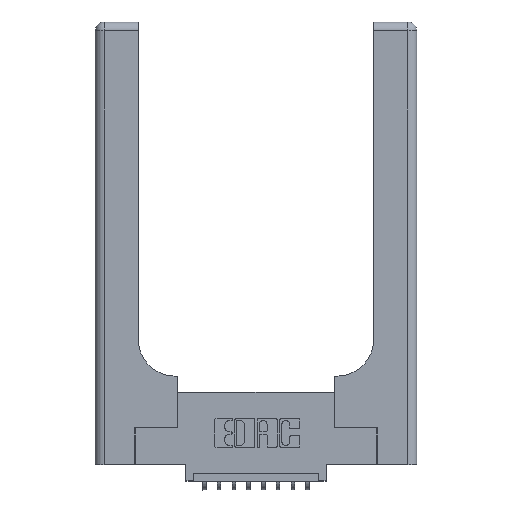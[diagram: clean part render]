
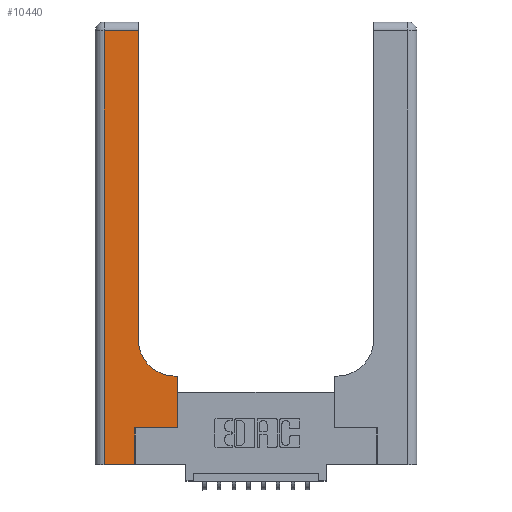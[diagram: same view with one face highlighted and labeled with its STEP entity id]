
A CAD part, top view. The second image highlights one B-rep face of the part: STEP entity #10440.
In plain terms, the highlighted planar face has unit normal (0, 0, 1).
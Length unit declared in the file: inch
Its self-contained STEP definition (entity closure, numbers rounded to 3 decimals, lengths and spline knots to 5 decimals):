
#51 = VECTOR ( 'NONE', #11838, 39.37008 ) ;
#222 = EDGE_CURVE ( 'NONE', #4829, #1192, #12432, .T. ) ;
#254 = CARTESIAN_POINT ( 'NONE',  ( 0.06, 2.94, 0.37 ) ) ;
#439 = DIRECTION ( 'NONE',  ( 0., 1., 0. ) ) ;
#472 = CIRCLE ( 'NONE', #12378, 0.25 ) ;
#584 = CARTESIAN_POINT ( 'NONE',  ( 0.269, 0.25, 0.37 ) ) ;
#1157 = ORIENTED_EDGE ( 'NONE', *, *, #15149, .T. ) ;
#1192 = VERTEX_POINT ( 'NONE', #12642 ) ;
#1278 = CARTESIAN_POINT ( 'NONE',  ( 0.269, 0., 0.37 ) ) ;
#1284 = VERTEX_POINT ( 'NONE', #8290 ) ;
#1441 = EDGE_CURVE ( 'NONE', #3802, #15325, #15326, .T. ) ;
#1727 = LINE ( 'NONE', #5273, #5572 ) ;
#1786 = CARTESIAN_POINT ( 'NONE',  ( 0.2915, 0.6, 0.37 ) ) ;
#1810 = EDGE_LOOP ( 'NONE', ( #11015, #13624, #15594, #1157, #11578, #8491, #12550, #9555, #2173 ) ) ;
#2173 = ORIENTED_EDGE ( 'NONE', *, *, #15000, .T. ) ;
#2683 = CARTESIAN_POINT ( 'NONE',  ( 0., 2.94, 0.37 ) ) ;
#2693 = VERTEX_POINT ( 'NONE', #13958 ) ;
#2738 = LINE ( 'NONE', #6694, #3914 ) ;
#3179 = CARTESIAN_POINT ( 'NONE',  ( 0., 3., 0.37 ) ) ;
#3290 = DIRECTION ( 'NONE',  ( 0., 0., -1. ) ) ;
#3368 = EDGE_CURVE ( 'NONE', #10573, #2693, #1727, .T. ) ;
#3802 = VERTEX_POINT ( 'NONE', #5037 ) ;
#3914 = VECTOR ( 'NONE', #10444, 39.37008 ) ;
#4421 = CARTESIAN_POINT ( 'NONE',  ( 0.269, 0.25, 0.37 ) ) ;
#4829 = VERTEX_POINT ( 'NONE', #12621 ) ;
#5037 = CARTESIAN_POINT ( 'NONE',  ( 0.269, 0., 0.37 ) ) ;
#5053 = DIRECTION ( 'NONE',  ( 1., 0., 0. ) ) ;
#5105 = VERTEX_POINT ( 'NONE', #10748 ) ;
#5273 = CARTESIAN_POINT ( 'NONE',  ( 0.2915, 3., 0.37 ) ) ;
#5572 = VECTOR ( 'NONE', #439, 39.37008 ) ;
#5710 = PLANE ( 'NONE',  #12329 ) ;
#5715 = EDGE_CURVE ( 'NONE', #13805, #1284, #6087, .T. ) ;
#6087 = LINE ( 'NONE', #15152, #14642 ) ;
#6694 = CARTESIAN_POINT ( 'NONE',  ( 0., 0., 0.37 ) ) ;
#6814 = DIRECTION ( 'NONE',  ( 0., -1., 0. ) ) ;
#6876 = DIRECTION ( 'NONE',  ( -1., 0., 0. ) ) ;
#6938 = DIRECTION ( 'NONE',  ( -1., 0., 0. ) ) ;
#7748 = LINE ( 'NONE', #2683, #11850 ) ;
#8081 = CARTESIAN_POINT ( 'NONE',  ( 0.5585, 0.25, 0.37 ) ) ;
#8119 = FACE_OUTER_BOUND ( 'NONE', #1810, .T. ) ;
#8146 = VECTOR ( 'NONE', #13171, 39.37008 ) ;
#8290 = CARTESIAN_POINT ( 'NONE',  ( 0.06, 0., 0.37 ) ) ;
#8491 = ORIENTED_EDGE ( 'NONE', *, *, #14017, .T. ) ;
#8907 = CARTESIAN_POINT ( 'NONE',  ( 0.5415, 0.85, 0.37 ) ) ;
#9164 = DIRECTION ( 'NONE',  ( 1., 0., 0. ) ) ;
#9555 = ORIENTED_EDGE ( 'NONE', *, *, #14635, .T. ) ;
#10245 = EDGE_CURVE ( 'NONE', #2693, #13805, #7748, .T. ) ;
#10440 = ADVANCED_FACE ( 'NONE', ( #8119 ), #5710, .F. ) ;
#10444 = DIRECTION ( 'NONE',  ( 1., 0., 0. ) ) ;
#10489 = VECTOR ( 'NONE', #6938, 39.37008 ) ;
#10573 = VERTEX_POINT ( 'NONE', #14032 ) ;
#10748 = CARTESIAN_POINT ( 'NONE',  ( 0.5415, 0.6, 0.37 ) ) ;
#11015 = ORIENTED_EDGE ( 'NONE', *, *, #3368, .T. ) ;
#11578 = ORIENTED_EDGE ( 'NONE', *, *, #1441, .T. ) ;
#11838 = DIRECTION ( 'NONE',  ( 0., 1., 0. ) ) ;
#11850 = VECTOR ( 'NONE', #13732, 39.37008 ) ;
#12087 = VECTOR ( 'NONE', #9164, 39.37008 ) ;
#12329 = AXIS2_PLACEMENT_3D ( 'NONE', #3179, #3290, #6876 ) ;
#12378 = AXIS2_PLACEMENT_3D ( 'NONE', #8907, #12624, #5053 ) ;
#12432 = LINE ( 'NONE', #8081, #8146 ) ;
#12550 = ORIENTED_EDGE ( 'NONE', *, *, #222, .T. ) ;
#12621 = CARTESIAN_POINT ( 'NONE',  ( 0.5585, 0.25, 0.37 ) ) ;
#12624 = DIRECTION ( 'NONE',  ( 0., 0., -1. ) ) ;
#12642 = CARTESIAN_POINT ( 'NONE',  ( 0.5585, 0.6, 0.37 ) ) ;
#13171 = DIRECTION ( 'NONE',  ( 0., 1., 0. ) ) ;
#13243 = LINE ( 'NONE', #1786, #10489 ) ;
#13624 = ORIENTED_EDGE ( 'NONE', *, *, #10245, .T. ) ;
#13732 = DIRECTION ( 'NONE',  ( -1., 0., 0. ) ) ;
#13805 = VERTEX_POINT ( 'NONE', #254 ) ;
#13958 = CARTESIAN_POINT ( 'NONE',  ( 0.2915, 2.94, 0.37 ) ) ;
#14017 = EDGE_CURVE ( 'NONE', #15325, #4829, #14789, .T. ) ;
#14032 = CARTESIAN_POINT ( 'NONE',  ( 0.2915, 0.85, 0.37 ) ) ;
#14635 = EDGE_CURVE ( 'NONE', #1192, #5105, #13243, .T. ) ;
#14642 = VECTOR ( 'NONE', #6814, 39.37008 ) ;
#14789 = LINE ( 'NONE', #584, #12087 ) ;
#15000 = EDGE_CURVE ( 'NONE', #5105, #10573, #472, .T. ) ;
#15149 = EDGE_CURVE ( 'NONE', #1284, #3802, #2738, .T. ) ;
#15152 = CARTESIAN_POINT ( 'NONE',  ( 0.06, 3., 0.37 ) ) ;
#15325 = VERTEX_POINT ( 'NONE', #4421 ) ;
#15326 = LINE ( 'NONE', #1278, #51 ) ;
#15594 = ORIENTED_EDGE ( 'NONE', *, *, #5715, .T. ) ;
